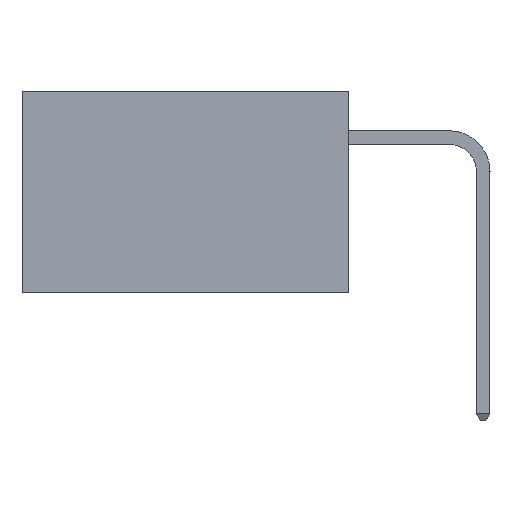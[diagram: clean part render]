
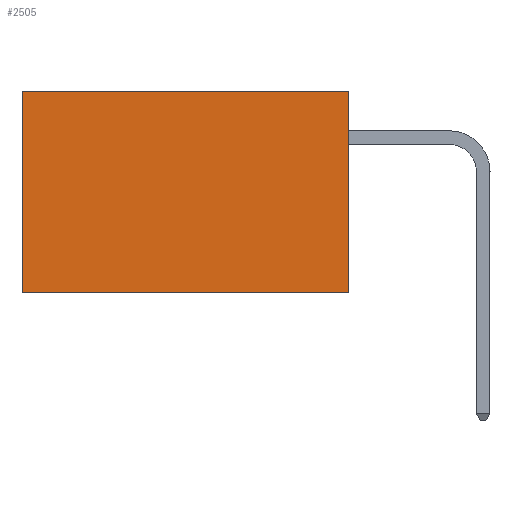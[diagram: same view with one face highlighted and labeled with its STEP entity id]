
A CAD part, left-side view. The second image highlights one B-rep face of the part: STEP entity #2505.
In plain terms, the highlighted planar face has unit normal (-1, 0, 0).
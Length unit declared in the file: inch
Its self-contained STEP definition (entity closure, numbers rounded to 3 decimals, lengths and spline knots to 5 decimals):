
#30 = LINE ( 'NONE', #13713, #16922 ) ;
#169 = CARTESIAN_POINT ( 'NONE',  ( 0.2875, 0., 0. ) ) ;
#344 = CARTESIAN_POINT ( 'NONE',  ( 0.2875, 0., 0. ) ) ;
#1200 = EDGE_CURVE ( 'NONE', #6406, #4258, #3399, .T. ) ;
#1282 = PLANE ( 'NONE',  #9355 ) ;
#2505 = ADVANCED_FACE ( 'NONE', ( #8248 ), #1282, .F. ) ;
#2981 = DIRECTION ( 'NONE',  ( 1., 0., 0. ) ) ;
#3270 = EDGE_CURVE ( 'NONE', #8550, #6406, #11740, .T. ) ;
#3353 = CARTESIAN_POINT ( 'NONE',  ( 0.2875, 0.6, -0.37 ) ) ;
#3399 = LINE ( 'NONE', #5430, #14094 ) ;
#4258 = VERTEX_POINT ( 'NONE', #3353 ) ;
#4581 = ORIENTED_EDGE ( 'NONE', *, *, #15075, .T. ) ;
#5118 = CARTESIAN_POINT ( 'NONE',  ( 0.2875, 0.6, 0. ) ) ;
#5430 = CARTESIAN_POINT ( 'NONE',  ( 0.2875, 0., -0.37 ) ) ;
#6406 = VERTEX_POINT ( 'NONE', #21070 ) ;
#7494 = EDGE_LOOP ( 'NONE', ( #9477, #16834, #18659, #4581 ) ) ;
#8248 = FACE_OUTER_BOUND ( 'NONE', #7494, .T. ) ;
#8550 = VERTEX_POINT ( 'NONE', #344 ) ;
#9039 = EDGE_CURVE ( 'NONE', #9177, #4258, #30, .T. ) ;
#9177 = VERTEX_POINT ( 'NONE', #5118 ) ;
#9299 = VECTOR ( 'NONE', #12172, 39.37008 ) ;
#9355 = AXIS2_PLACEMENT_3D ( 'NONE', #13242, #2981, #14949 ) ;
#9477 = ORIENTED_EDGE ( 'NONE', *, *, #9039, .T. ) ;
#11740 = LINE ( 'NONE', #169, #9299 ) ;
#12172 = DIRECTION ( 'NONE',  ( 0., 0., -1. ) ) ;
#13242 = CARTESIAN_POINT ( 'NONE',  ( 0.2875, 0., 0. ) ) ;
#13713 = CARTESIAN_POINT ( 'NONE',  ( 0.2875, 0.6, 0. ) ) ;
#14094 = VECTOR ( 'NONE', #19083, 39.37008 ) ;
#14949 = DIRECTION ( 'NONE',  ( 0., 0., -1. ) ) ;
#15075 = EDGE_CURVE ( 'NONE', #8550, #9177, #20782, .T. ) ;
#15608 = DIRECTION ( 'NONE',  ( 0., 0., -1. ) ) ;
#16834 = ORIENTED_EDGE ( 'NONE', *, *, #1200, .F. ) ;
#16922 = VECTOR ( 'NONE', #15608, 39.37008 ) ;
#17918 = DIRECTION ( 'NONE',  ( 0., 1., 0. ) ) ;
#18659 = ORIENTED_EDGE ( 'NONE', *, *, #3270, .F. ) ;
#19083 = DIRECTION ( 'NONE',  ( 0., 1., 0. ) ) ;
#19393 = CARTESIAN_POINT ( 'NONE',  ( 0.2875, 0., 0. ) ) ;
#19451 = VECTOR ( 'NONE', #17918, 39.37008 ) ;
#20782 = LINE ( 'NONE', #19393, #19451 ) ;
#21070 = CARTESIAN_POINT ( 'NONE',  ( 0.2875, 0., -0.37 ) ) ;
